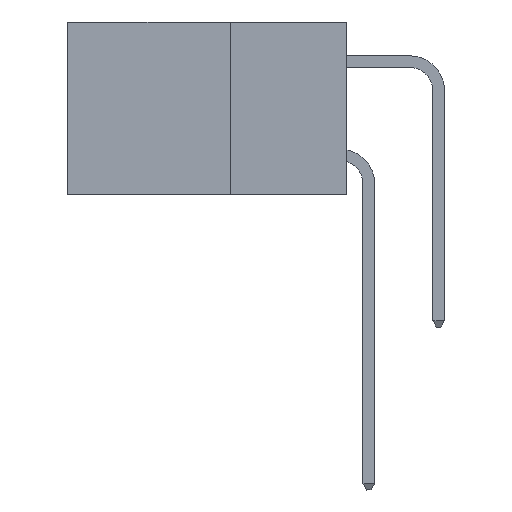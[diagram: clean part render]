
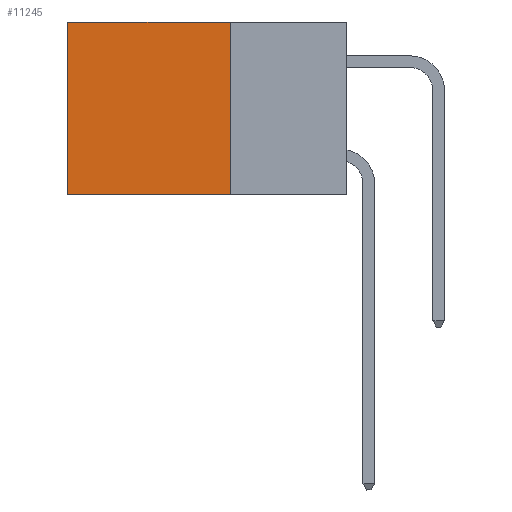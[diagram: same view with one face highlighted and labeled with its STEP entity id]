
A CAD part, left-side view. The second image highlights one B-rep face of the part: STEP entity #11245.
In plain terms, the highlighted planar face has unit normal (-1, 0, 0).
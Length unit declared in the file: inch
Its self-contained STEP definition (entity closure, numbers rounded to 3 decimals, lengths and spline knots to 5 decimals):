
#66 = VERTEX_POINT ( 'NONE', #169 ) ;
#169 = CARTESIAN_POINT ( 'NONE',  ( 0.2875, 0.25, -0.37 ) ) ;
#715 = FACE_OUTER_BOUND ( 'NONE', #8949, .T. ) ;
#896 = ORIENTED_EDGE ( 'NONE', *, *, #4814, .F. ) ;
#1053 = EDGE_CURVE ( 'NONE', #7511, #6957, #6987, .T. ) ;
#1662 = EDGE_CURVE ( 'NONE', #6957, #2519, #10003, .T. ) ;
#1859 = DIRECTION ( 'NONE',  ( 0., 1., 0. ) ) ;
#1873 = ORIENTED_EDGE ( 'NONE', *, *, #1053, .T. ) ;
#2351 = DIRECTION ( 'NONE',  ( 0., 1., 0. ) ) ;
#2477 = VECTOR ( 'NONE', #2351, 39.37008 ) ;
#2519 = VERTEX_POINT ( 'NONE', #12488 ) ;
#2837 = CARTESIAN_POINT ( 'NONE',  ( 0.2875, 0.25, -0.37 ) ) ;
#2895 = AXIS2_PLACEMENT_3D ( 'NONE', #12726, #2916, #3057 ) ;
#2916 = DIRECTION ( 'NONE',  ( 1., 0., 0. ) ) ;
#3057 = DIRECTION ( 'NONE',  ( 0., 0., -1. ) ) ;
#3172 = CARTESIAN_POINT ( 'NONE',  ( 0.2875, 0.25, 0. ) ) ;
#3731 = CARTESIAN_POINT ( 'NONE',  ( 0.2875, 0.6, 0. ) ) ;
#4814 = EDGE_CURVE ( 'NONE', #66, #2519, #8532, .T. ) ;
#5231 = DIRECTION ( 'NONE',  ( 0., 0., -1. ) ) ;
#6415 = VECTOR ( 'NONE', #5231, 39.37008 ) ;
#6465 = CARTESIAN_POINT ( 'NONE',  ( 0.2875, 0.25, 0. ) ) ;
#6937 = CARTESIAN_POINT ( 'NONE',  ( 0.2875, 0.25, 0. ) ) ;
#6957 = VERTEX_POINT ( 'NONE', #10105 ) ;
#6987 = LINE ( 'NONE', #6465, #2477 ) ;
#7511 = VERTEX_POINT ( 'NONE', #6937 ) ;
#7955 = ORIENTED_EDGE ( 'NONE', *, *, #1662, .T. ) ;
#8532 = LINE ( 'NONE', #2837, #10224 ) ;
#8544 = ORIENTED_EDGE ( 'NONE', *, *, #11315, .F. ) ;
#8949 = EDGE_LOOP ( 'NONE', ( #7955, #896, #8544, #1873 ) ) ;
#9477 = PLANE ( 'NONE',  #2895 ) ;
#10003 = LINE ( 'NONE', #3731, #11479 ) ;
#10105 = CARTESIAN_POINT ( 'NONE',  ( 0.2875, 0.6, 0. ) ) ;
#10224 = VECTOR ( 'NONE', #1859, 39.37008 ) ;
#11245 = ADVANCED_FACE ( 'NONE', ( #715 ), #9477, .F. ) ;
#11315 = EDGE_CURVE ( 'NONE', #7511, #66, #11421, .T. ) ;
#11421 = LINE ( 'NONE', #3172, #6415 ) ;
#11479 = VECTOR ( 'NONE', #13372, 39.37008 ) ;
#12488 = CARTESIAN_POINT ( 'NONE',  ( 0.2875, 0.6, -0.37 ) ) ;
#12726 = CARTESIAN_POINT ( 'NONE',  ( 0.2875, 0.25, 0. ) ) ;
#13372 = DIRECTION ( 'NONE',  ( 0., 0., -1. ) ) ;
